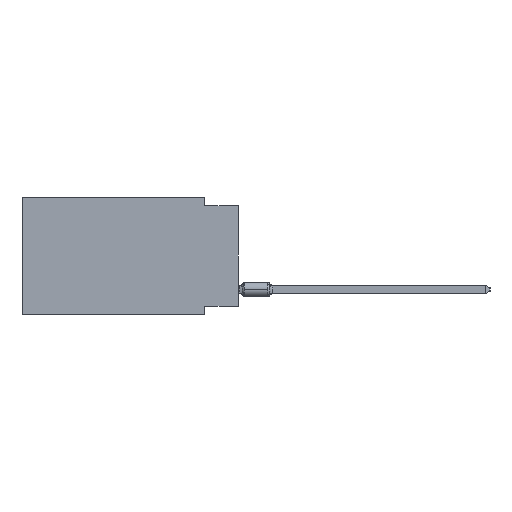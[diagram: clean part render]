
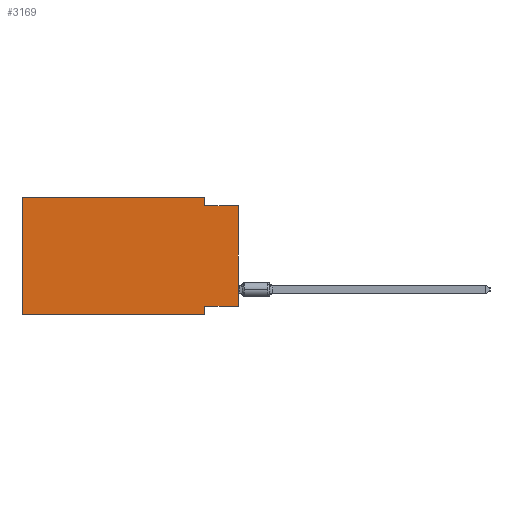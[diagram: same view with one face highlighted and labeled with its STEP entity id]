
A CAD part, left-side view. The second image highlights one B-rep face of the part: STEP entity #3169.
In plain terms, the highlighted planar face has unit normal (-1, 0, 0).
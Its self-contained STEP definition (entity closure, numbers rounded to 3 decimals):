
#403 = DIRECTION ( 'NONE',  ( 0., 0., -1. ) ) ;
#1328 = ORIENTED_EDGE ( 'NONE', *, *, #23687, .T. ) ;
#1701 = VECTOR ( 'NONE', #403, 1000. ) ;
#1965 = ORIENTED_EDGE ( 'NONE', *, *, #39383, .F. ) ;
#2184 = VERTEX_POINT ( 'NONE', #23986 ) ;
#3169 = ADVANCED_FACE ( 'NONE', ( #16310 ), #42737, .F. ) ;
#3283 = DIRECTION ( 'NONE',  ( 1., 0., 0. ) ) ;
#3480 = CARTESIAN_POINT ( 'NONE',  ( 0., 16.383, 0. ) ) ;
#3750 = LINE ( 'NONE', #27171, #14886 ) ;
#5227 = CARTESIAN_POINT ( 'NONE',  ( 0., 0., -8.255 ) ) ;
#6135 = CARTESIAN_POINT ( 'NONE',  ( 0., 16.383, -8.89 ) ) ;
#6273 = VECTOR ( 'NONE', #33384, 1000. ) ;
#6415 = VERTEX_POINT ( 'NONE', #41633 ) ;
#6947 = LINE ( 'NONE', #11052, #6273 ) ;
#7674 = DIRECTION ( 'NONE',  ( 0., -1., 0. ) ) ;
#7921 = ORIENTED_EDGE ( 'NONE', *, *, #37674, .F. ) ;
#8078 = CARTESIAN_POINT ( 'NONE',  ( 0., 0., -8.255 ) ) ;
#8702 = VERTEX_POINT ( 'NONE', #36798 ) ;
#11052 = CARTESIAN_POINT ( 'NONE',  ( 0., 0., 0. ) ) ;
#11942 = VERTEX_POINT ( 'NONE', #42247 ) ;
#12221 = ORIENTED_EDGE ( 'NONE', *, *, #16496, .F. ) ;
#12980 = ORIENTED_EDGE ( 'NONE', *, *, #37200, .F. ) ;
#14886 = VECTOR ( 'NONE', #36264, 1000. ) ;
#15843 = LINE ( 'NONE', #5227, #21431 ) ;
#16310 = FACE_OUTER_BOUND ( 'NONE', #28883, .T. ) ;
#16496 = EDGE_CURVE ( 'NONE', #2184, #41740, #32969, .T. ) ;
#18816 = VERTEX_POINT ( 'NONE', #25663 ) ;
#20362 = VECTOR ( 'NONE', #38659, 1000. ) ;
#20393 = DIRECTION ( 'NONE',  ( 0., -1., 0. ) ) ;
#20595 = AXIS2_PLACEMENT_3D ( 'NONE', #39055, #3283, #39483 ) ;
#20610 = ORIENTED_EDGE ( 'NONE', *, *, #27324, .F. ) ;
#21431 = VECTOR ( 'NONE', #35557, 1000. ) ;
#22125 = EDGE_CURVE ( 'NONE', #35978, #6415, #23700, .T. ) ;
#22220 = ORIENTED_EDGE ( 'NONE', *, *, #38019, .T. ) ;
#23474 = VERTEX_POINT ( 'NONE', #8078 ) ;
#23687 = EDGE_CURVE ( 'NONE', #23474, #6415, #6947, .T. ) ;
#23700 = LINE ( 'NONE', #24574, #31164 ) ;
#23986 = CARTESIAN_POINT ( 'NONE',  ( 0., 16.383, 0. ) ) ;
#24470 = LINE ( 'NONE', #34207, #1701 ) ;
#24574 = CARTESIAN_POINT ( 'NONE',  ( 0., 0., -0.635 ) ) ;
#25663 = CARTESIAN_POINT ( 'NONE',  ( 0., 2.54, -8.89 ) ) ;
#27171 = CARTESIAN_POINT ( 'NONE',  ( 0., 16.383, 0. ) ) ;
#27324 = EDGE_CURVE ( 'NONE', #23474, #8702, #15843, .T. ) ;
#28497 = LINE ( 'NONE', #6135, #20362 ) ;
#28883 = EDGE_LOOP ( 'NONE', ( #1328, #38451, #12980, #12221, #1965, #22220, #7921, #20610 ) ) ;
#29769 = CARTESIAN_POINT ( 'NONE',  ( 0., 2.54, -8.89 ) ) ;
#31164 = VECTOR ( 'NONE', #7674, 1000. ) ;
#31514 = VECTOR ( 'NONE', #32368, 1000. ) ;
#32368 = DIRECTION ( 'NONE',  ( 0., 0., -1. ) ) ;
#32969 = LINE ( 'NONE', #3480, #38099 ) ;
#33384 = DIRECTION ( 'NONE',  ( 0., 0., 1. ) ) ;
#34207 = CARTESIAN_POINT ( 'NONE',  ( 0., 2.54, 0. ) ) ;
#35557 = DIRECTION ( 'NONE',  ( 0., 1., 0. ) ) ;
#35978 = VERTEX_POINT ( 'NONE', #37224 ) ;
#36264 = DIRECTION ( 'NONE',  ( 0., 0., 1. ) ) ;
#36795 = CARTESIAN_POINT ( 'NONE',  ( 0., 2.54, 0. ) ) ;
#36798 = CARTESIAN_POINT ( 'NONE',  ( 0., 2.54, -8.255 ) ) ;
#37200 = EDGE_CURVE ( 'NONE', #41740, #35978, #24470, .T. ) ;
#37224 = CARTESIAN_POINT ( 'NONE',  ( 0., 2.54, -0.635 ) ) ;
#37674 = EDGE_CURVE ( 'NONE', #8702, #18816, #39294, .T. ) ;
#38019 = EDGE_CURVE ( 'NONE', #11942, #18816, #28497, .T. ) ;
#38099 = VECTOR ( 'NONE', #20393, 1000. ) ;
#38451 = ORIENTED_EDGE ( 'NONE', *, *, #22125, .F. ) ;
#38659 = DIRECTION ( 'NONE',  ( 0., -1., 0. ) ) ;
#39055 = CARTESIAN_POINT ( 'NONE',  ( 0., 16.383, 0. ) ) ;
#39294 = LINE ( 'NONE', #29769, #31514 ) ;
#39383 = EDGE_CURVE ( 'NONE', #11942, #2184, #3750, .T. ) ;
#39483 = DIRECTION ( 'NONE',  ( 0., 0., -1. ) ) ;
#41633 = CARTESIAN_POINT ( 'NONE',  ( 0., 0., -0.635 ) ) ;
#41740 = VERTEX_POINT ( 'NONE', #36795 ) ;
#42247 = CARTESIAN_POINT ( 'NONE',  ( 0., 16.383, -8.89 ) ) ;
#42737 = PLANE ( 'NONE',  #20595 ) ;
